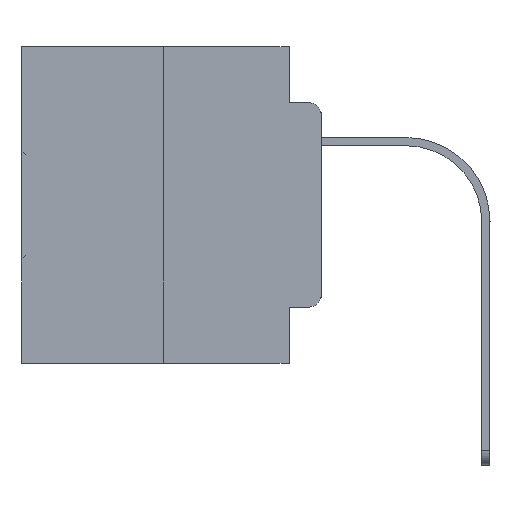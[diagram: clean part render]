
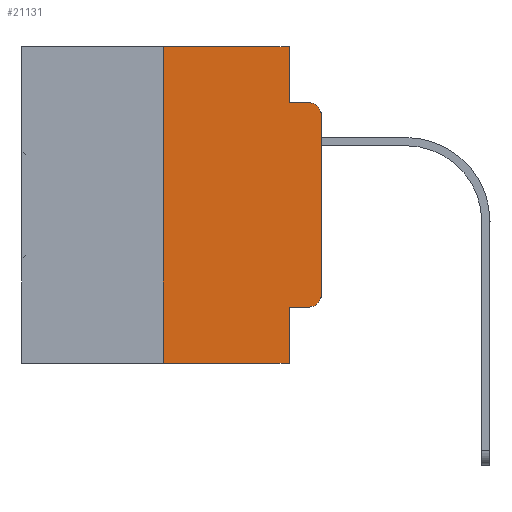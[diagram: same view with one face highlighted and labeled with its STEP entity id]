
A CAD part, left-side view. The second image highlights one B-rep face of the part: STEP entity #21131.
In plain terms, the highlighted planar face has unit normal (-1, 0, 0).
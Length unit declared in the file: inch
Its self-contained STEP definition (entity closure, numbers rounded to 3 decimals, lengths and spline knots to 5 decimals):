
#420 = VECTOR ( 'NONE', #30028, 39.37008 ) ;
#486 = ORIENTED_EDGE ( 'NONE', *, *, #1428, .T. ) ;
#810 = CARTESIAN_POINT ( 'NONE',  ( 0., 0., 0. ) ) ;
#838 = VECTOR ( 'NONE', #26266, 39.37008 ) ;
#942 = VERTEX_POINT ( 'NONE', #18973 ) ;
#1428 = EDGE_CURVE ( 'NONE', #942, #21648, #29072, .T. ) ;
#1836 = LINE ( 'NONE', #32126, #22520 ) ;
#1916 = ORIENTED_EDGE ( 'NONE', *, *, #26155, .F. ) ;
#3030 = VECTOR ( 'NONE', #27333, 39.37008 ) ;
#5464 = CARTESIAN_POINT ( 'NONE',  ( 0., 0.02, -0.3915 ) ) ;
#5505 = VERTEX_POINT ( 'NONE', #22327 ) ;
#5676 = AXIS2_PLACEMENT_3D ( 'NONE', #13934, #23413, #13588 ) ;
#5846 = LINE ( 'NONE', #810, #11043 ) ;
#6151 = DIRECTION ( 'NONE',  ( 0., 0., -1. ) ) ;
#6766 = CARTESIAN_POINT ( 'NONE',  ( 0., 0.051, -0.0885 ) ) ;
#7047 = DIRECTION ( 'NONE',  ( 0., 0., -1. ) ) ;
#7049 = CARTESIAN_POINT ( 'NONE',  ( 0., 0.473, 0. ) ) ;
#7193 = CARTESIAN_POINT ( 'NONE',  ( 0., 0.473, 0. ) ) ;
#7195 = ORIENTED_EDGE ( 'NONE', *, *, #8008, .T. ) ;
#8008 = EDGE_CURVE ( 'NONE', #23702, #10234, #23766, .T. ) ;
#8130 = DIRECTION ( 'NONE',  ( -1., 0., 0. ) ) ;
#8763 = EDGE_CURVE ( 'NONE', #10234, #24372, #5846, .T. ) ;
#8928 = EDGE_CURVE ( 'NONE', #942, #22093, #32451, .T. ) ;
#9039 = LINE ( 'NONE', #7049, #3030 ) ;
#9174 = DIRECTION ( 'NONE',  ( 0., 0., 1. ) ) ;
#9769 = CARTESIAN_POINT ( 'NONE',  ( 0., 0.051, -0.0885 ) ) ;
#10106 = CARTESIAN_POINT ( 'NONE',  ( 0., 0., -0.3915 ) ) ;
#10181 = VECTOR ( 'NONE', #6151, 39.37008 ) ;
#10234 = VERTEX_POINT ( 'NONE', #10106 ) ;
#11043 = VECTOR ( 'NONE', #31441, 39.37008 ) ;
#11051 = EDGE_CURVE ( 'NONE', #5505, #23702, #1836, .T. ) ;
#11069 = VECTOR ( 'NONE', #9174, 39.37008 ) ;
#11570 = AXIS2_PLACEMENT_3D ( 'NONE', #5464, #8130, #25909 ) ;
#12565 = CARTESIAN_POINT ( 'NONE',  ( 0., 0., -0.1085 ) ) ;
#13588 = DIRECTION ( 'NONE',  ( 0., 0., -1. ) ) ;
#13622 = CARTESIAN_POINT ( 'NONE',  ( 0., 0.02, -0.4115 ) ) ;
#13708 = VERTEX_POINT ( 'NONE', #19171 ) ;
#13934 = CARTESIAN_POINT ( 'NONE',  ( 0., 0.02, -0.1085 ) ) ;
#14150 = ORIENTED_EDGE ( 'NONE', *, *, #11051, .T. ) ;
#14179 = VERTEX_POINT ( 'NONE', #29959 ) ;
#14493 = CARTESIAN_POINT ( 'NONE',  ( 0., 0.25, 0. ) ) ;
#14494 = VERTEX_POINT ( 'NONE', #6766 ) ;
#14857 = DIRECTION ( 'NONE',  ( 0., -1., 0. ) ) ;
#15428 = ORIENTED_EDGE ( 'NONE', *, *, #8928, .F. ) ;
#16535 = ORIENTED_EDGE ( 'NONE', *, *, #19094, .F. ) ;
#17060 = LINE ( 'NONE', #19209, #20116 ) ;
#18787 = CARTESIAN_POINT ( 'NONE',  ( 0., 0.473, -0.5 ) ) ;
#18973 = CARTESIAN_POINT ( 'NONE',  ( 0., 0.25, -0.5 ) ) ;
#19094 = EDGE_CURVE ( 'NONE', #14494, #13708, #32544, .T. ) ;
#19171 = CARTESIAN_POINT ( 'NONE',  ( 0., 0.02, -0.0885 ) ) ;
#19209 = CARTESIAN_POINT ( 'NONE',  ( 0., 0.051, 0. ) ) ;
#20116 = VECTOR ( 'NONE', #31644, 39.37008 ) ;
#21131 = ADVANCED_FACE ( 'NONE', ( #22489 ), #22328, .F. ) ;
#21297 = CARTESIAN_POINT ( 'NONE',  ( 0., 0.051, 0. ) ) ;
#21438 = EDGE_CURVE ( 'NONE', #5505, #21648, #23614, .T. ) ;
#21648 = VERTEX_POINT ( 'NONE', #29933 ) ;
#22093 = VERTEX_POINT ( 'NONE', #25332 ) ;
#22147 = DIRECTION ( 'NONE',  ( 1., 0., 0. ) ) ;
#22327 = CARTESIAN_POINT ( 'NONE',  ( 0., 0.051, -0.4115 ) ) ;
#22328 = PLANE ( 'NONE',  #22371 ) ;
#22371 = AXIS2_PLACEMENT_3D ( 'NONE', #7193, #22147, #7047 ) ;
#22489 = FACE_OUTER_BOUND ( 'NONE', #23963, .T. ) ;
#22520 = VECTOR ( 'NONE', #14857, 39.37008 ) ;
#23413 = DIRECTION ( 'NONE',  ( -1., 0., 0. ) ) ;
#23614 = LINE ( 'NONE', #21297, #10181 ) ;
#23702 = VERTEX_POINT ( 'NONE', #13622 ) ;
#23766 = CIRCLE ( 'NONE', #11570, 0.02 ) ;
#23963 = EDGE_LOOP ( 'NONE', ( #28069, #32089, #16535, #24377, #1916, #15428, #486, #31139, #14150, #7195 ) ) ;
#24261 = CIRCLE ( 'NONE', #5676, 0.02 ) ;
#24372 = VERTEX_POINT ( 'NONE', #12565 ) ;
#24377 = ORIENTED_EDGE ( 'NONE', *, *, #24706, .F. ) ;
#24706 = EDGE_CURVE ( 'NONE', #14179, #14494, #17060, .T. ) ;
#25332 = CARTESIAN_POINT ( 'NONE',  ( 0., 0.25, 0. ) ) ;
#25457 = EDGE_CURVE ( 'NONE', #24372, #13708, #24261, .T. ) ;
#25909 = DIRECTION ( 'NONE',  ( 0., 0., -1. ) ) ;
#26155 = EDGE_CURVE ( 'NONE', #22093, #14179, #9039, .T. ) ;
#26266 = DIRECTION ( 'NONE',  ( 0., -1., 0. ) ) ;
#27333 = DIRECTION ( 'NONE',  ( 0., -1., 0. ) ) ;
#28069 = ORIENTED_EDGE ( 'NONE', *, *, #8763, .T. ) ;
#29072 = LINE ( 'NONE', #18787, #838 ) ;
#29933 = CARTESIAN_POINT ( 'NONE',  ( 0., 0.051, -0.5 ) ) ;
#29959 = CARTESIAN_POINT ( 'NONE',  ( 0., 0.051, 0. ) ) ;
#30028 = DIRECTION ( 'NONE',  ( 0., -1., 0. ) ) ;
#31139 = ORIENTED_EDGE ( 'NONE', *, *, #21438, .F. ) ;
#31441 = DIRECTION ( 'NONE',  ( 0., 0., 1. ) ) ;
#31644 = DIRECTION ( 'NONE',  ( 0., 0., -1. ) ) ;
#32089 = ORIENTED_EDGE ( 'NONE', *, *, #25457, .T. ) ;
#32126 = CARTESIAN_POINT ( 'NONE',  ( 0., 0.051, -0.4115 ) ) ;
#32451 = LINE ( 'NONE', #14493, #11069 ) ;
#32544 = LINE ( 'NONE', #9769, #420 ) ;
